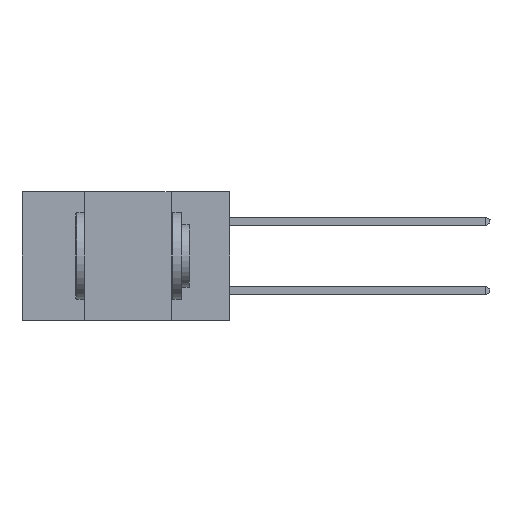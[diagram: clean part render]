
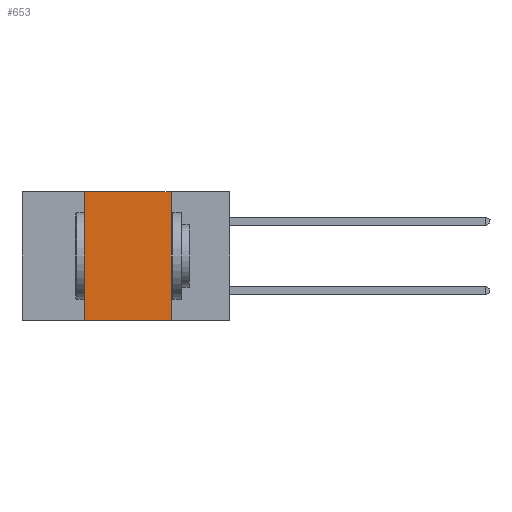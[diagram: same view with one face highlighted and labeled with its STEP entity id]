
A CAD part, left-side view. The second image highlights one B-rep face of the part: STEP entity #653.
In plain terms, the highlighted planar face has unit normal (-1, 0, 0).
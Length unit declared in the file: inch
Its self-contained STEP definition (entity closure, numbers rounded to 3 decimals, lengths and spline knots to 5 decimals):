
#653 = ADVANCED_FACE ( 'NONE', ( #18070 ), #17346, .F. ) ;
#757 = LINE ( 'NONE', #796, #22651 ) ;
#796 = CARTESIAN_POINT ( 'NONE',  ( 0., 0.6, -0.37 ) ) ;
#1186 = DIRECTION ( 'NONE',  ( 1., 0., 0. ) ) ;
#2968 = DIRECTION ( 'NONE',  ( 0., 0., -1. ) ) ;
#3435 = DIRECTION ( 'NONE',  ( 0., -1., 0. ) ) ;
#4366 = VERTEX_POINT ( 'NONE', #8537 ) ;
#4896 = EDGE_LOOP ( 'NONE', ( #15730, #11213, #22932, #10487 ) ) ;
#5664 = LINE ( 'NONE', #5911, #8235 ) ;
#5888 = VERTEX_POINT ( 'NONE', #9833 ) ;
#5911 = CARTESIAN_POINT ( 'NONE',  ( 0., 0.42, 0. ) ) ;
#7371 = VECTOR ( 'NONE', #10436, 39.37008 ) ;
#7875 = EDGE_CURVE ( 'NONE', #11741, #16476, #10835, .T. ) ;
#7949 = LINE ( 'NONE', #20681, #20301 ) ;
#8175 = CARTESIAN_POINT ( 'NONE',  ( 0., 0.17, 0. ) ) ;
#8235 = VECTOR ( 'NONE', #12754, 39.37008 ) ;
#8537 = CARTESIAN_POINT ( 'NONE',  ( 0., 0.17, -0.37 ) ) ;
#9670 = CARTESIAN_POINT ( 'NONE',  ( 0., 0.42, 0. ) ) ;
#9833 = CARTESIAN_POINT ( 'NONE',  ( 0., 0.42, -0.37 ) ) ;
#10265 = CARTESIAN_POINT ( 'NONE',  ( 0., 0.6, 0. ) ) ;
#10436 = DIRECTION ( 'NONE',  ( 0., -1., 0. ) ) ;
#10487 = ORIENTED_EDGE ( 'NONE', *, *, #24735, .T. ) ;
#10835 = LINE ( 'NONE', #10265, #7371 ) ;
#11213 = ORIENTED_EDGE ( 'NONE', *, *, #7875, .F. ) ;
#11741 = VERTEX_POINT ( 'NONE', #9670 ) ;
#12754 = DIRECTION ( 'NONE',  ( 0., 0., 1. ) ) ;
#14031 = AXIS2_PLACEMENT_3D ( 'NONE', #15323, #1186, #2968 ) ;
#14500 = EDGE_CURVE ( 'NONE', #5888, #11741, #5664, .T. ) ;
#15323 = CARTESIAN_POINT ( 'NONE',  ( 0., 0.6, 0. ) ) ;
#15730 = ORIENTED_EDGE ( 'NONE', *, *, #20865, .F. ) ;
#16476 = VERTEX_POINT ( 'NONE', #8175 ) ;
#17346 = PLANE ( 'NONE',  #14031 ) ;
#18070 = FACE_OUTER_BOUND ( 'NONE', #4896, .T. ) ;
#20301 = VECTOR ( 'NONE', #24674, 39.37008 ) ;
#20681 = CARTESIAN_POINT ( 'NONE',  ( 0., 0.17, 0. ) ) ;
#20865 = EDGE_CURVE ( 'NONE', #16476, #4366, #7949, .T. ) ;
#22651 = VECTOR ( 'NONE', #3435, 39.37008 ) ;
#22932 = ORIENTED_EDGE ( 'NONE', *, *, #14500, .F. ) ;
#24674 = DIRECTION ( 'NONE',  ( 0., 0., -1. ) ) ;
#24735 = EDGE_CURVE ( 'NONE', #5888, #4366, #757, .T. ) ;
